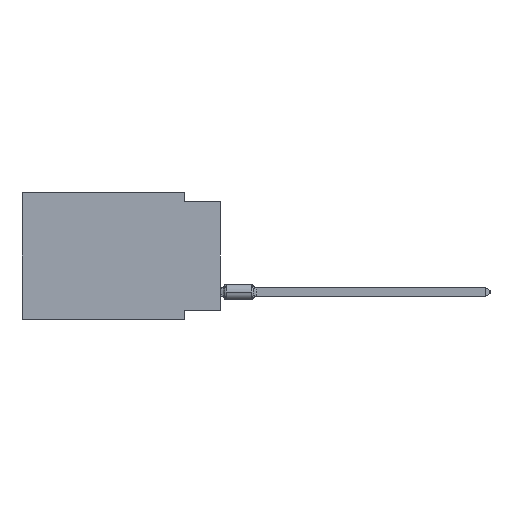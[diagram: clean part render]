
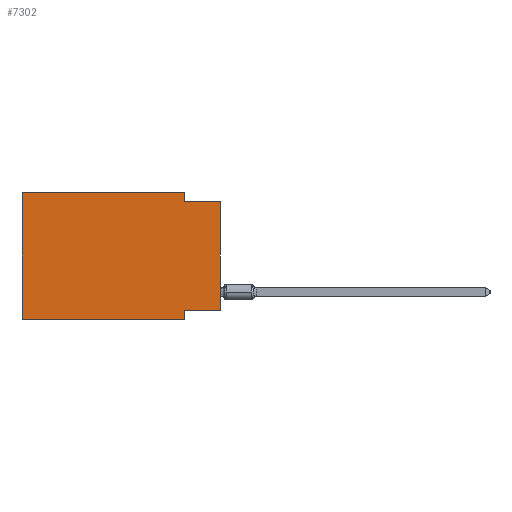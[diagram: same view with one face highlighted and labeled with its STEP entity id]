
A CAD part, left-side view. The second image highlights one B-rep face of the part: STEP entity #7302.
In plain terms, the highlighted planar face has unit normal (-1, 0, 0).
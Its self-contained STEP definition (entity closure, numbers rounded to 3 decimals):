
#205 = EDGE_CURVE ( 'NONE', #21667, #5787, #36891, .T. ) ;
#275 = CARTESIAN_POINT ( 'NONE',  ( 0., 2.54, -8.255 ) ) ;
#732 = ORIENTED_EDGE ( 'NONE', *, *, #205, .F. ) ;
#969 = VECTOR ( 'NONE', #16890, 1000. ) ;
#1050 = EDGE_CURVE ( 'NONE', #5472, #35990, #6467, .T. ) ;
#1280 = VECTOR ( 'NONE', #7275, 1000. ) ;
#1311 = DIRECTION ( 'NONE',  ( 0., -1., 0. ) ) ;
#1631 = LINE ( 'NONE', #16492, #1280 ) ;
#2956 = CARTESIAN_POINT ( 'NONE',  ( 0., 2.54, -8.89 ) ) ;
#3023 = ORIENTED_EDGE ( 'NONE', *, *, #16113, .F. ) ;
#4644 = EDGE_CURVE ( 'NONE', #35990, #28858, #1631, .T. ) ;
#5148 = EDGE_CURVE ( 'NONE', #36284, #29493, #5551, .T. ) ;
#5472 = VERTEX_POINT ( 'NONE', #37840 ) ;
#5551 = LINE ( 'NONE', #17594, #28824 ) ;
#5787 = VERTEX_POINT ( 'NONE', #13919 ) ;
#6467 = LINE ( 'NONE', #34373, #19053 ) ;
#7275 = DIRECTION ( 'NONE',  ( 0., -1., 0. ) ) ;
#7302 = ADVANCED_FACE ( 'NONE', ( #31544 ), #32144, .F. ) ;
#10789 = CARTESIAN_POINT ( 'NONE',  ( 0., 2.54, 0. ) ) ;
#10983 = LINE ( 'NONE', #10789, #14900 ) ;
#13919 = CARTESIAN_POINT ( 'NONE',  ( 0., 2.54, -8.89 ) ) ;
#14900 = VECTOR ( 'NONE', #38709, 1000. ) ;
#15161 = DIRECTION ( 'NONE',  ( 0., 0., 1. ) ) ;
#15195 = DIRECTION ( 'NONE',  ( 0., 0., -1. ) ) ;
#16113 = EDGE_CURVE ( 'NONE', #29401, #29493, #25994, .T. ) ;
#16492 = CARTESIAN_POINT ( 'NONE',  ( 0., 13.97, 0. ) ) ;
#16890 = DIRECTION ( 'NONE',  ( 0., -1., 0. ) ) ;
#16923 = CARTESIAN_POINT ( 'NONE',  ( 0., 0., -8.255 ) ) ;
#17594 = CARTESIAN_POINT ( 'NONE',  ( 0., 0., 0. ) ) ;
#18167 = EDGE_LOOP ( 'NONE', ( #32140, #3023, #37426, #31622, #38367, #19663, #732, #22108 ) ) ;
#19053 = VECTOR ( 'NONE', #30735, 1000. ) ;
#19663 = ORIENTED_EDGE ( 'NONE', *, *, #32115, .T. ) ;
#19778 = CARTESIAN_POINT ( 'NONE',  ( 0., 0., -8.255 ) ) ;
#20301 = LINE ( 'NONE', #38596, #969 ) ;
#21415 = VECTOR ( 'NONE', #28616, 1000. ) ;
#21667 = VERTEX_POINT ( 'NONE', #275 ) ;
#22108 = ORIENTED_EDGE ( 'NONE', *, *, #35786, .F. ) ;
#22509 = DIRECTION ( 'NONE',  ( 1., 0., 0. ) ) ;
#22716 = DIRECTION ( 'NONE',  ( 0., 0., -1. ) ) ;
#23316 = VECTOR ( 'NONE', #1311, 1000. ) ;
#23756 = AXIS2_PLACEMENT_3D ( 'NONE', #35167, #22509, #22716 ) ;
#23760 = EDGE_CURVE ( 'NONE', #28858, #29401, #10983, .T. ) ;
#25135 = CARTESIAN_POINT ( 'NONE',  ( 0., 2.54, -0.635 ) ) ;
#25994 = LINE ( 'NONE', #35230, #23316 ) ;
#28616 = DIRECTION ( 'NONE',  ( 0., 1., 0. ) ) ;
#28824 = VECTOR ( 'NONE', #15161, 1000. ) ;
#28858 = VERTEX_POINT ( 'NONE', #34087 ) ;
#29401 = VERTEX_POINT ( 'NONE', #25135 ) ;
#29493 = VERTEX_POINT ( 'NONE', #32368 ) ;
#30735 = DIRECTION ( 'NONE',  ( 0., 0., 1. ) ) ;
#31544 = FACE_OUTER_BOUND ( 'NONE', #18167, .T. ) ;
#31622 = ORIENTED_EDGE ( 'NONE', *, *, #4644, .F. ) ;
#32115 = EDGE_CURVE ( 'NONE', #5472, #5787, #20301, .T. ) ;
#32140 = ORIENTED_EDGE ( 'NONE', *, *, #5148, .T. ) ;
#32144 = PLANE ( 'NONE',  #23756 ) ;
#32368 = CARTESIAN_POINT ( 'NONE',  ( 0., 0., -0.635 ) ) ;
#32998 = VECTOR ( 'NONE', #15195, 1000. ) ;
#33423 = CARTESIAN_POINT ( 'NONE',  ( 0., 13.97, 0. ) ) ;
#34087 = CARTESIAN_POINT ( 'NONE',  ( 0., 2.54, 0. ) ) ;
#34373 = CARTESIAN_POINT ( 'NONE',  ( 0., 13.97, 0. ) ) ;
#35167 = CARTESIAN_POINT ( 'NONE',  ( 0., 13.97, 0. ) ) ;
#35230 = CARTESIAN_POINT ( 'NONE',  ( 0., 0., -0.635 ) ) ;
#35786 = EDGE_CURVE ( 'NONE', #36284, #21667, #37677, .T. ) ;
#35990 = VERTEX_POINT ( 'NONE', #33423 ) ;
#36284 = VERTEX_POINT ( 'NONE', #16923 ) ;
#36891 = LINE ( 'NONE', #2956, #32998 ) ;
#37426 = ORIENTED_EDGE ( 'NONE', *, *, #23760, .F. ) ;
#37677 = LINE ( 'NONE', #19778, #21415 ) ;
#37840 = CARTESIAN_POINT ( 'NONE',  ( 0., 13.97, -8.89 ) ) ;
#38367 = ORIENTED_EDGE ( 'NONE', *, *, #1050, .F. ) ;
#38596 = CARTESIAN_POINT ( 'NONE',  ( 0., 13.97, -8.89 ) ) ;
#38709 = DIRECTION ( 'NONE',  ( 0., 0., -1. ) ) ;
